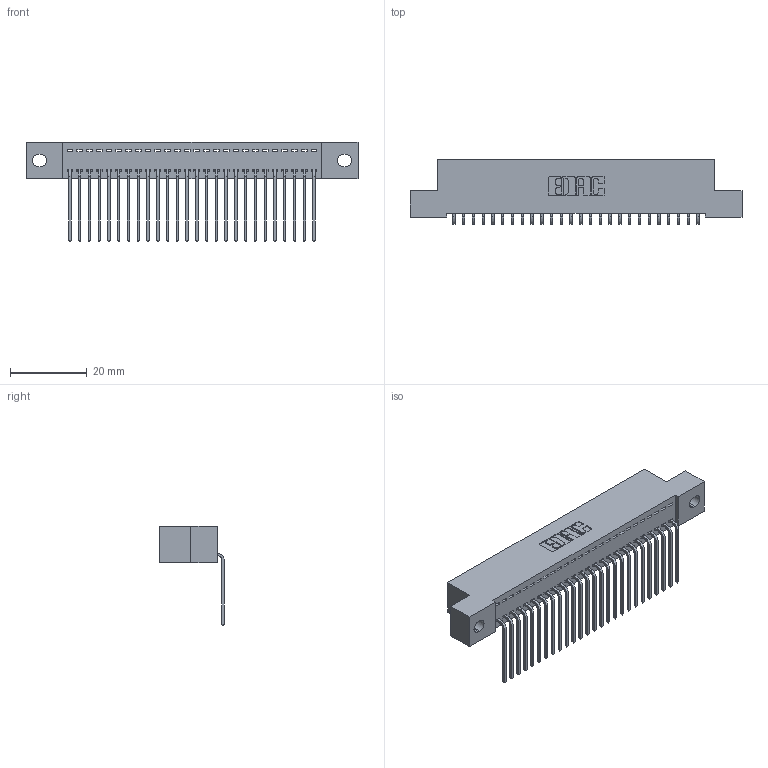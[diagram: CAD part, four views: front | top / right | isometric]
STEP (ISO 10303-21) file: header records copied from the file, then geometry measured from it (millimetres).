
FILE_DESCRIPTION (( 'STEP AP203' ), '1' );
FILE_NAME ('392-026-559-102.STEP', '2018-08-15T20:11:29', ( '' ), ( '' ), 'SwSTEP 2.0', 'SolidWorks 2016', '' );
FILE_SCHEMA (( 'CONFIG_CONTROL_DESIGN' ));
Length unit declared in the file: inch
Products named in the file (3): 342 Part_.128 Slot; 345-292-001_558 559 Tail - 1; 392-026-559-102
Assembly tree (27 placements, depth 2):
  392-026-559-102
    342 Part_.128 Slot
    345-292-001_558 559 Tail - 1  x26
Bounding box: 86.36 x 16.83 x 25.78 mm (x, y, z)
Volume: 7547.6 mm3; surface area: 11036.2 mm2
Topology: 27 solids, 27 shells, 1674 faces, 5043 edges, 3326 vertices
Faces by surface type: plane 1214, cylinder 460
Entity records: 18051 total; most frequent: CARTESIAN_POINT 3124, ORIENTED_EDGE 3086, DIRECTION 2667, EDGE_CURVE 1543, VECTOR 1415, LINE 1415, VERTEX_POINT 1026, AXIS2_PLACEMENT_3D 626
